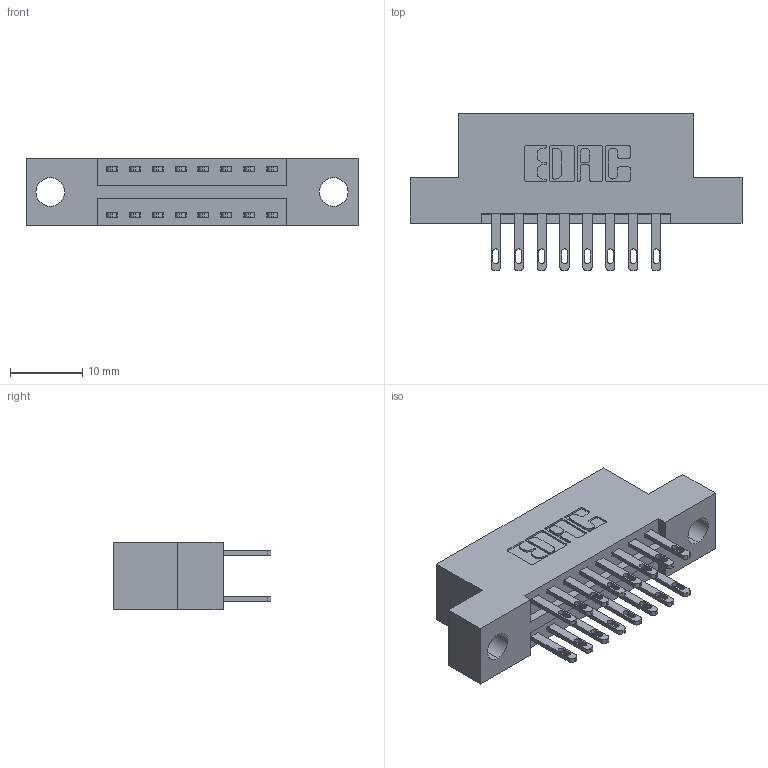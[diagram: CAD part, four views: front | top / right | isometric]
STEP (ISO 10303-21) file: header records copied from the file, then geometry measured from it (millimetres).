
FILE_DESCRIPTION (( 'STEP AP203' ), '1' );
FILE_NAME ('346-016-500-204.STEP', '2022-05-18T15:13:28', ( '' ), ( '' ), 'SwSTEP 2.0', 'SolidWorks 2020', '' );
FILE_SCHEMA (( 'CONFIG_CONTROL_DESIGN' ));
Length unit declared in the file: inch
Products named in the file (3): 346 Part_Flush Mounting Lugs - 0.156 Dia-TH; 346-016-500-204; 345-292-001_345-293-100
Assembly tree (17 placements, depth 2):
  346-016-500-204
    346 Part_Flush Mounting Lugs - 0.156 Dia-TH
    345-292-001_345-293-100  x16
Bounding box: 45.97 x 21.84 x 9.4 mm (x, y, z)
Volume: 4161.9 mm3; surface area: 5201.8 mm2
Topology: 17 solids, 17 shells, 904 faces, 2717 edges, 1810 vertices
Faces by surface type: plane 554, cylinder 350
Entity records: 10147 total; most frequent: CARTESIAN_POINT 1722, ORIENTED_EDGE 1654, DIRECTION 1571, EDGE_CURVE 827, VECTOR 659, LINE 659, VERTEX_POINT 550, AXIS2_PLACEMENT_3D 456
